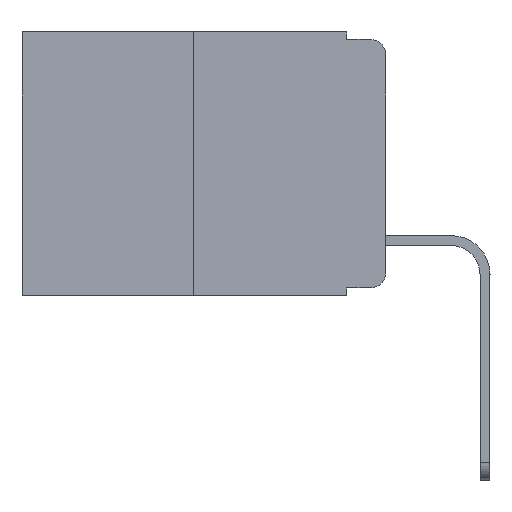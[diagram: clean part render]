
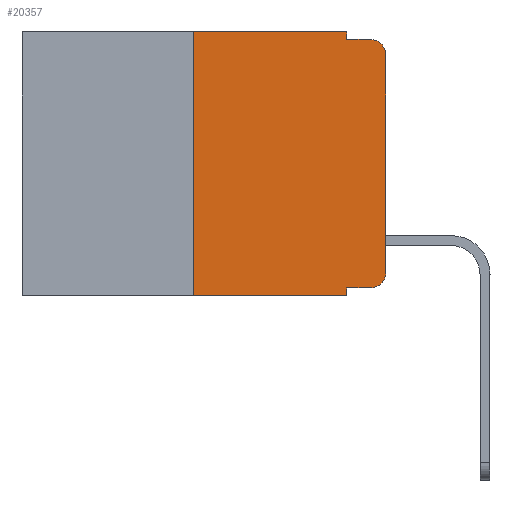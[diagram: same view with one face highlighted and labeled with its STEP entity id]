
A CAD part, left-side view. The second image highlights one B-rep face of the part: STEP entity #20357.
In plain terms, the highlighted planar face has unit normal (-1, 0, 0).
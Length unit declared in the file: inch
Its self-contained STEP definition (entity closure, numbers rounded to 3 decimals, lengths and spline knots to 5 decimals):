
#347 = LINE ( 'NONE', #9799, #5983 ) ;
#654 = ORIENTED_EDGE ( 'NONE', *, *, #20837, .F. ) ;
#963 = CARTESIAN_POINT ( 'NONE',  ( 0., 0.473, -0.343 ) ) ;
#1329 = DIRECTION ( 'NONE',  ( 0., 0., 1. ) ) ;
#1656 = CARTESIAN_POINT ( 'NONE',  ( 0., 0.051, 0. ) ) ;
#1756 = ORIENTED_EDGE ( 'NONE', *, *, #5305, .T. ) ;
#1783 = AXIS2_PLACEMENT_3D ( 'NONE', #14568, #19317, #12868 ) ;
#2131 = VERTEX_POINT ( 'NONE', #18372 ) ;
#2161 = VERTEX_POINT ( 'NONE', #8342 ) ;
#2418 = DIRECTION ( 'NONE',  ( 0., -1., 0. ) ) ;
#2500 = LINE ( 'NONE', #16420, #15003 ) ;
#2593 = DIRECTION ( 'NONE',  ( -1., 0., 0. ) ) ;
#3161 = ORIENTED_EDGE ( 'NONE', *, *, #19011, .T. ) ;
#3388 = EDGE_CURVE ( 'NONE', #5603, #17463, #7741, .T. ) ;
#3743 = EDGE_CURVE ( 'NONE', #2161, #10575, #17653, .T. ) ;
#3926 = ORIENTED_EDGE ( 'NONE', *, *, #3388, .F. ) ;
#4922 = AXIS2_PLACEMENT_3D ( 'NONE', #12209, #17155, #17294 ) ;
#5260 = CARTESIAN_POINT ( 'NONE',  ( 0., 0.25, 0. ) ) ;
#5305 = EDGE_CURVE ( 'NONE', #2161, #18852, #8430, .T. ) ;
#5493 = AXIS2_PLACEMENT_3D ( 'NONE', #15709, #2593, #15640 ) ;
#5603 = VERTEX_POINT ( 'NONE', #1656 ) ;
#5983 = VECTOR ( 'NONE', #16256, 39.37008 ) ;
#6235 = FACE_OUTER_BOUND ( 'NONE', #7862, .T. ) ;
#6715 = VECTOR ( 'NONE', #12415, 39.37008 ) ;
#7492 = CARTESIAN_POINT ( 'NONE',  ( 0., 0.02, -0.01 ) ) ;
#7741 = LINE ( 'NONE', #12560, #6715 ) ;
#7862 = EDGE_LOOP ( 'NONE', ( #16492, #10255, #9049, #3926, #18602, #654, #20065, #15397, #1756, #3161 ) ) ;
#7960 = PLANE ( 'NONE',  #1783 ) ;
#8235 = LINE ( 'NONE', #963, #12573 ) ;
#8342 = CARTESIAN_POINT ( 'NONE',  ( 0., 0.051, -0.333 ) ) ;
#8349 = EDGE_CURVE ( 'NONE', #2131, #10575, #8235, .T. ) ;
#8430 = LINE ( 'NONE', #15151, #13508 ) ;
#9049 = ORIENTED_EDGE ( 'NONE', *, *, #10800, .F. ) ;
#9544 = CARTESIAN_POINT ( 'NONE',  ( 0., 0., 0. ) ) ;
#9667 = EDGE_CURVE ( 'NONE', #16293, #19314, #15258, .T. ) ;
#9799 = CARTESIAN_POINT ( 'NONE',  ( 0., 0.473, 0. ) ) ;
#9818 = CARTESIAN_POINT ( 'NONE',  ( 0., 0., -0.313 ) ) ;
#10255 = ORIENTED_EDGE ( 'NONE', *, *, #20213, .T. ) ;
#10456 = DIRECTION ( 'NONE',  ( 0., 0., -1. ) ) ;
#10560 = CIRCLE ( 'NONE', #5493, 0.02 ) ;
#10575 = VERTEX_POINT ( 'NONE', #20693 ) ;
#10800 = EDGE_CURVE ( 'NONE', #17463, #17170, #2500, .T. ) ;
#11553 = LINE ( 'NONE', #5260, #16379 ) ;
#12107 = DIRECTION ( 'NONE',  ( 0., -1., 0. ) ) ;
#12209 = CARTESIAN_POINT ( 'NONE',  ( 0., 0.02, -0.313 ) ) ;
#12415 = DIRECTION ( 'NONE',  ( 0., 0., -1. ) ) ;
#12560 = CARTESIAN_POINT ( 'NONE',  ( 0., 0.051, 0. ) ) ;
#12573 = VECTOR ( 'NONE', #2418, 39.37008 ) ;
#12868 = DIRECTION ( 'NONE',  ( 0., 0., -1. ) ) ;
#13508 = VECTOR ( 'NONE', #12107, 39.37008 ) ;
#13604 = CARTESIAN_POINT ( 'NONE',  ( 0., 0.051, 0. ) ) ;
#14568 = CARTESIAN_POINT ( 'NONE',  ( 0., 0.473, 0. ) ) ;
#14690 = CIRCLE ( 'NONE', #4922, 0.02 ) ;
#14874 = DIRECTION ( 'NONE',  ( 0., -1., 0. ) ) ;
#15003 = VECTOR ( 'NONE', #14874, 39.37008 ) ;
#15151 = CARTESIAN_POINT ( 'NONE',  ( 0., 0.051, -0.333 ) ) ;
#15252 = VERTEX_POINT ( 'NONE', #16796 ) ;
#15258 = LINE ( 'NONE', #9544, #15524 ) ;
#15397 = ORIENTED_EDGE ( 'NONE', *, *, #3743, .F. ) ;
#15524 = VECTOR ( 'NONE', #1329, 39.37008 ) ;
#15640 = DIRECTION ( 'NONE',  ( 0., 0., -1. ) ) ;
#15709 = CARTESIAN_POINT ( 'NONE',  ( 0., 0.02, -0.03 ) ) ;
#16256 = DIRECTION ( 'NONE',  ( 0., -1., 0. ) ) ;
#16293 = VERTEX_POINT ( 'NONE', #9818 ) ;
#16379 = VECTOR ( 'NONE', #18284, 39.37008 ) ;
#16420 = CARTESIAN_POINT ( 'NONE',  ( 0., 0.051, -0.01 ) ) ;
#16492 = ORIENTED_EDGE ( 'NONE', *, *, #9667, .T. ) ;
#16796 = CARTESIAN_POINT ( 'NONE',  ( 0., 0.25, 0. ) ) ;
#17155 = DIRECTION ( 'NONE',  ( -1., 0., 0. ) ) ;
#17170 = VERTEX_POINT ( 'NONE', #7492 ) ;
#17294 = DIRECTION ( 'NONE',  ( 0., 0., -1. ) ) ;
#17375 = VECTOR ( 'NONE', #10456, 39.37008 ) ;
#17463 = VERTEX_POINT ( 'NONE', #19434 ) ;
#17653 = LINE ( 'NONE', #13604, #17375 ) ;
#18284 = DIRECTION ( 'NONE',  ( 0., 0., 1. ) ) ;
#18372 = CARTESIAN_POINT ( 'NONE',  ( 0., 0.25, -0.343 ) ) ;
#18602 = ORIENTED_EDGE ( 'NONE', *, *, #20447, .F. ) ;
#18852 = VERTEX_POINT ( 'NONE', #20026 ) ;
#19011 = EDGE_CURVE ( 'NONE', #18852, #16293, #14690, .T. ) ;
#19314 = VERTEX_POINT ( 'NONE', #19650 ) ;
#19317 = DIRECTION ( 'NONE',  ( 1., 0., 0. ) ) ;
#19434 = CARTESIAN_POINT ( 'NONE',  ( 0., 0.051, -0.01 ) ) ;
#19650 = CARTESIAN_POINT ( 'NONE',  ( 0., 0., -0.03 ) ) ;
#20026 = CARTESIAN_POINT ( 'NONE',  ( 0., 0.02, -0.333 ) ) ;
#20065 = ORIENTED_EDGE ( 'NONE', *, *, #8349, .T. ) ;
#20213 = EDGE_CURVE ( 'NONE', #19314, #17170, #10560, .T. ) ;
#20357 = ADVANCED_FACE ( 'NONE', ( #6235 ), #7960, .F. ) ;
#20447 = EDGE_CURVE ( 'NONE', #15252, #5603, #347, .T. ) ;
#20693 = CARTESIAN_POINT ( 'NONE',  ( 0., 0.051, -0.343 ) ) ;
#20837 = EDGE_CURVE ( 'NONE', #2131, #15252, #11553, .T. ) ;
